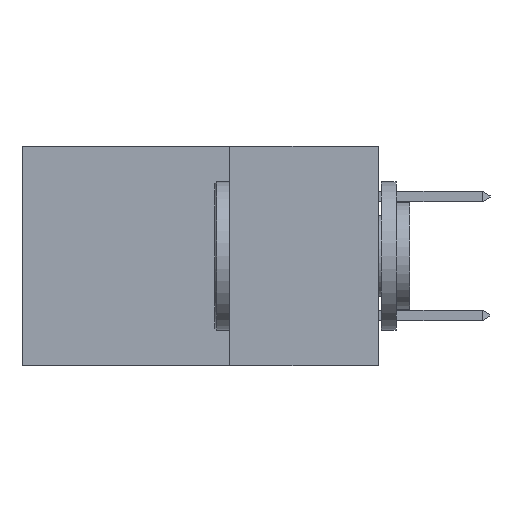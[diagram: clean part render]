
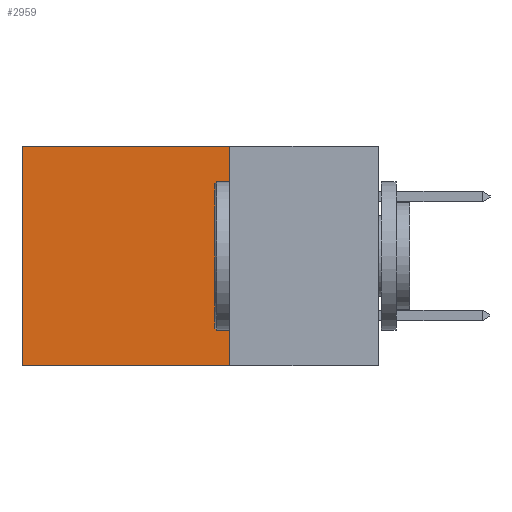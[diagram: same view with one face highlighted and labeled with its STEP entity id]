
A CAD part, left-side view. The second image highlights one B-rep face of the part: STEP entity #2959.
In plain terms, the highlighted planar face has unit normal (-1, 0, 0).
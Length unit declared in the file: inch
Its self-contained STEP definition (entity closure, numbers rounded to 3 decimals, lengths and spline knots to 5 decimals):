
#274 = EDGE_CURVE ( 'NONE', #4213, #2026, #10461, .T. ) ;
#444 = ORIENTED_EDGE ( 'NONE', *, *, #22293, .F. ) ;
#884 = DIRECTION ( 'NONE',  ( 0., 0., -1. ) ) ;
#1349 = EDGE_LOOP ( 'NONE', ( #9280, #15054, #444, #13537 ) ) ;
#1696 = LINE ( 'NONE', #5271, #10689 ) ;
#2026 = VERTEX_POINT ( 'NONE', #15038 ) ;
#2959 = ADVANCED_FACE ( 'NONE', ( #14125 ), #13770, .F. ) ;
#3030 = LINE ( 'NONE', #13520, #16770 ) ;
#4114 = VERTEX_POINT ( 'NONE', #19701 ) ;
#4213 = VERTEX_POINT ( 'NONE', #5779 ) ;
#5271 = CARTESIAN_POINT ( 'NONE',  ( 0.2615, 0.6, -0.37 ) ) ;
#5357 = DIRECTION ( 'NONE',  ( 0., 0., -1. ) ) ;
#5767 = VECTOR ( 'NONE', #21006, 39.37008 ) ;
#5779 = CARTESIAN_POINT ( 'NONE',  ( 0.2615, 0.25, -0.37 ) ) ;
#5908 = VERTEX_POINT ( 'NONE', #18384 ) ;
#7517 = EDGE_CURVE ( 'NONE', #5908, #2026, #1696, .T. ) ;
#9280 = ORIENTED_EDGE ( 'NONE', *, *, #7517, .T. ) ;
#9479 = CARTESIAN_POINT ( 'NONE',  ( 0.2615, 0.25, 0. ) ) ;
#10461 = LINE ( 'NONE', #16954, #5767 ) ;
#10689 = VECTOR ( 'NONE', #5357, 39.37008 ) ;
#11690 = AXIS2_PLACEMENT_3D ( 'NONE', #13188, #13087, #13037 ) ;
#13037 = DIRECTION ( 'NONE',  ( 0., 0., -1. ) ) ;
#13087 = DIRECTION ( 'NONE',  ( 1., 0., 0. ) ) ;
#13138 = EDGE_CURVE ( 'NONE', #4114, #5908, #16372, .T. ) ;
#13188 = CARTESIAN_POINT ( 'NONE',  ( 0.2615, 0.25, -0.37 ) ) ;
#13520 = CARTESIAN_POINT ( 'NONE',  ( 0.2615, 0.25, -0.37 ) ) ;
#13537 = ORIENTED_EDGE ( 'NONE', *, *, #13138, .T. ) ;
#13770 = PLANE ( 'NONE',  #11690 ) ;
#14125 = FACE_OUTER_BOUND ( 'NONE', #1349, .T. ) ;
#15038 = CARTESIAN_POINT ( 'NONE',  ( 0.2615, 0.6, -0.37 ) ) ;
#15054 = ORIENTED_EDGE ( 'NONE', *, *, #274, .F. ) ;
#16372 = LINE ( 'NONE', #9479, #16922 ) ;
#16770 = VECTOR ( 'NONE', #884, 39.37008 ) ;
#16922 = VECTOR ( 'NONE', #21914, 39.37008 ) ;
#16954 = CARTESIAN_POINT ( 'NONE',  ( 0.2615, 0.25, -0.37 ) ) ;
#18384 = CARTESIAN_POINT ( 'NONE',  ( 0.2615, 0.6, 0. ) ) ;
#19701 = CARTESIAN_POINT ( 'NONE',  ( 0.2615, 0.25, 0. ) ) ;
#21006 = DIRECTION ( 'NONE',  ( 0., 1., 0. ) ) ;
#21914 = DIRECTION ( 'NONE',  ( 0., 1., 0. ) ) ;
#22293 = EDGE_CURVE ( 'NONE', #4114, #4213, #3030, .T. ) ;
